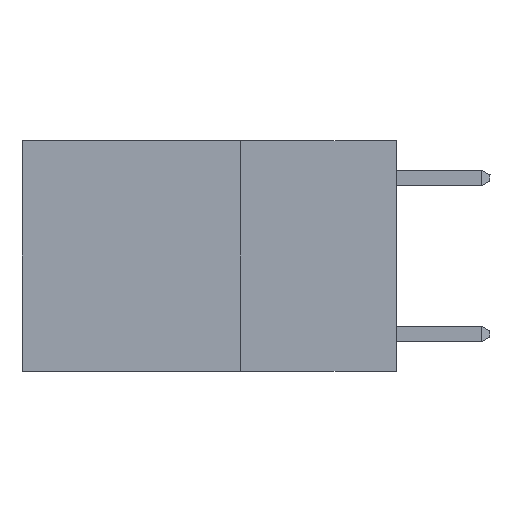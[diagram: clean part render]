
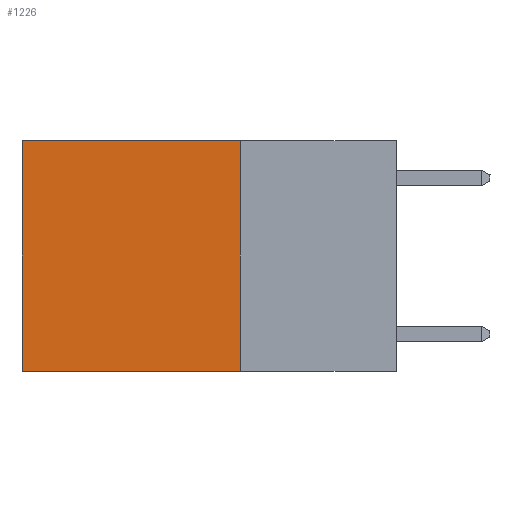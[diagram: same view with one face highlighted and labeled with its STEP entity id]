
A CAD part, left-side view. The second image highlights one B-rep face of the part: STEP entity #1226.
In plain terms, the highlighted planar face has unit normal (-1, 0, 0).
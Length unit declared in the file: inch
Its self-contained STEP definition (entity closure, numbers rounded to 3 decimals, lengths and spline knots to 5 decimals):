
#283 = VECTOR ( 'NONE', #815, 39.37008 ) ;
#461 = DIRECTION ( 'NONE',  ( 0., 1., 0. ) ) ;
#496 = LINE ( 'NONE', #888, #283 ) ;
#518 = LINE ( 'NONE', #1104, #604 ) ;
#604 = VECTOR ( 'NONE', #1159, 39.37008 ) ;
#660 = VERTEX_POINT ( 'NONE', #8753 ) ;
#690 = CARTESIAN_POINT ( 'NONE',  ( 0.2625, 0.25, 0. ) ) ;
#740 = CARTESIAN_POINT ( 'NONE',  ( 0.2625, 0.25, -0.37 ) ) ;
#815 = DIRECTION ( 'NONE',  ( 0., 0., -1. ) ) ;
#888 = CARTESIAN_POINT ( 'NONE',  ( 0.2625, 0.25, 0. ) ) ;
#1104 = CARTESIAN_POINT ( 'NONE',  ( 0.2625, 0.25, -0.37 ) ) ;
#1159 = DIRECTION ( 'NONE',  ( 0., 1., 0. ) ) ;
#1226 = ADVANCED_FACE ( 'NONE', ( #2226 ), #4505, .F. ) ;
#1538 = EDGE_CURVE ( 'NONE', #1601, #660, #518, .T. ) ;
#1589 = EDGE_CURVE ( 'NONE', #4232, #1601, #496, .T. ) ;
#1601 = VERTEX_POINT ( 'NONE', #740 ) ;
#2007 = EDGE_LOOP ( 'NONE', ( #7545, #7681, #7707, #7752 ) ) ;
#2226 = FACE_OUTER_BOUND ( 'NONE', #2007, .T. ) ;
#2273 = EDGE_CURVE ( 'NONE', #4232, #7438, #7133, .T. ) ;
#3086 = CARTESIAN_POINT ( 'NONE',  ( 0.2625, 0.25, 0. ) ) ;
#3186 = LINE ( 'NONE', #8465, #5008 ) ;
#4218 = DIRECTION ( 'NONE',  ( 0., 0., -1. ) ) ;
#4231 = DIRECTION ( 'NONE',  ( 1., 0., 0. ) ) ;
#4232 = VERTEX_POINT ( 'NONE', #3086 ) ;
#4313 = CARTESIAN_POINT ( 'NONE',  ( 0.2625, 0.25, 0. ) ) ;
#4505 = PLANE ( 'NONE',  #7011 ) ;
#5008 = VECTOR ( 'NONE', #8532, 39.37008 ) ;
#6054 = CARTESIAN_POINT ( 'NONE',  ( 0.2625, 0.6, 0. ) ) ;
#6715 = EDGE_CURVE ( 'NONE', #7438, #660, #3186, .T. ) ;
#7011 = AXIS2_PLACEMENT_3D ( 'NONE', #4313, #4231, #4218 ) ;
#7133 = LINE ( 'NONE', #690, #7328 ) ;
#7328 = VECTOR ( 'NONE', #461, 39.37008 ) ;
#7438 = VERTEX_POINT ( 'NONE', #6054 ) ;
#7545 = ORIENTED_EDGE ( 'NONE', *, *, #6715, .T. ) ;
#7681 = ORIENTED_EDGE ( 'NONE', *, *, #1538, .F. ) ;
#7707 = ORIENTED_EDGE ( 'NONE', *, *, #1589, .F. ) ;
#7752 = ORIENTED_EDGE ( 'NONE', *, *, #2273, .T. ) ;
#8465 = CARTESIAN_POINT ( 'NONE',  ( 0.2625, 0.6, 0. ) ) ;
#8532 = DIRECTION ( 'NONE',  ( 0., 0., -1. ) ) ;
#8753 = CARTESIAN_POINT ( 'NONE',  ( 0.2625, 0.6, -0.37 ) ) ;
